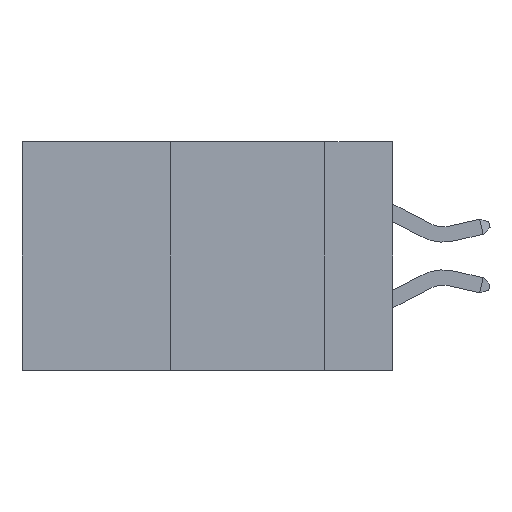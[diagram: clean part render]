
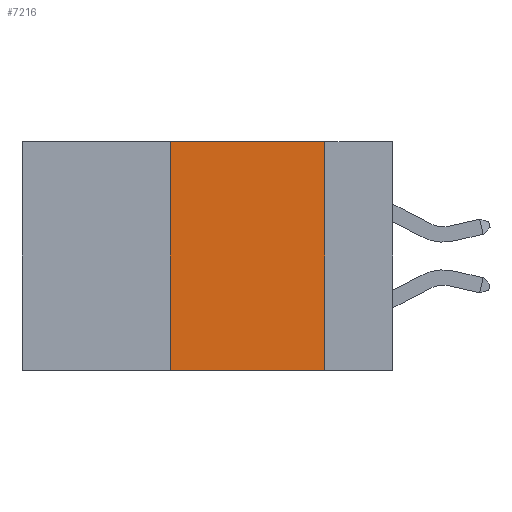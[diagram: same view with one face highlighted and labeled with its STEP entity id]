
A CAD part, left-side view. The second image highlights one B-rep face of the part: STEP entity #7216.
In plain terms, the highlighted planar face has unit normal (-1, 0, 0).
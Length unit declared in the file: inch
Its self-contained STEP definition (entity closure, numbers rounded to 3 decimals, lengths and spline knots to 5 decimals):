
#915 = FACE_OUTER_BOUND ( 'NONE', #4220, .T. ) ;
#1119 = ORIENTED_EDGE ( 'NONE', *, *, #30496, .F. ) ;
#2266 = VERTEX_POINT ( 'NONE', #2293 ) ;
#2293 = CARTESIAN_POINT ( 'NONE',  ( 0., 0.11, 0. ) ) ;
#3966 = CARTESIAN_POINT ( 'NONE',  ( 0., 0.6, 0. ) ) ;
#4220 = EDGE_LOOP ( 'NONE', ( #1119, #17563, #8876, #30420 ) ) ;
#4413 = VERTEX_POINT ( 'NONE', #17421 ) ;
#6650 = DIRECTION ( 'NONE',  ( 1., 0., 0. ) ) ;
#7216 = ADVANCED_FACE ( 'NONE', ( #915 ), #32798, .F. ) ;
#7852 = CARTESIAN_POINT ( 'NONE',  ( 0., 0.6, 0. ) ) ;
#8070 = DIRECTION ( 'NONE',  ( 0., -1., 0. ) ) ;
#8876 = ORIENTED_EDGE ( 'NONE', *, *, #10263, .F. ) ;
#10263 = EDGE_CURVE ( 'NONE', #23681, #4413, #28654, .T. ) ;
#10290 = EDGE_CURVE ( 'NONE', #4413, #2266, #22755, .T. ) ;
#12297 = AXIS2_PLACEMENT_3D ( 'NONE', #3966, #6650, #27260 ) ;
#12434 = VECTOR ( 'NONE', #25042, 39.37008 ) ;
#17421 = CARTESIAN_POINT ( 'NONE',  ( 0., 0.36, 0. ) ) ;
#17563 = ORIENTED_EDGE ( 'NONE', *, *, #10290, .F. ) ;
#22258 = CARTESIAN_POINT ( 'NONE',  ( 0., 0.36, -0.37 ) ) ;
#22406 = LINE ( 'NONE', #30984, #29024 ) ;
#22755 = LINE ( 'NONE', #7852, #12434 ) ;
#23681 = VERTEX_POINT ( 'NONE', #22258 ) ;
#25042 = DIRECTION ( 'NONE',  ( 0., -1., 0. ) ) ;
#25425 = DIRECTION ( 'NONE',  ( 0., 0., 1. ) ) ;
#25527 = DIRECTION ( 'NONE',  ( 0., 0., -1. ) ) ;
#25614 = CARTESIAN_POINT ( 'NONE',  ( 0., 0.36, 0. ) ) ;
#25917 = VERTEX_POINT ( 'NONE', #36073 ) ;
#25931 = VECTOR ( 'NONE', #25527, 39.37008 ) ;
#26271 = CARTESIAN_POINT ( 'NONE',  ( 0., 0.11, 0. ) ) ;
#27260 = DIRECTION ( 'NONE',  ( 0., 0., -1. ) ) ;
#28654 = LINE ( 'NONE', #25614, #35563 ) ;
#29024 = VECTOR ( 'NONE', #8070, 39.37008 ) ;
#30420 = ORIENTED_EDGE ( 'NONE', *, *, #31450, .T. ) ;
#30496 = EDGE_CURVE ( 'NONE', #2266, #25917, #31234, .T. ) ;
#30984 = CARTESIAN_POINT ( 'NONE',  ( 0., 0.6, -0.37 ) ) ;
#31234 = LINE ( 'NONE', #26271, #25931 ) ;
#31450 = EDGE_CURVE ( 'NONE', #23681, #25917, #22406, .T. ) ;
#32798 = PLANE ( 'NONE',  #12297 ) ;
#35563 = VECTOR ( 'NONE', #25425, 39.37008 ) ;
#36073 = CARTESIAN_POINT ( 'NONE',  ( 0., 0.11, -0.37 ) ) ;
